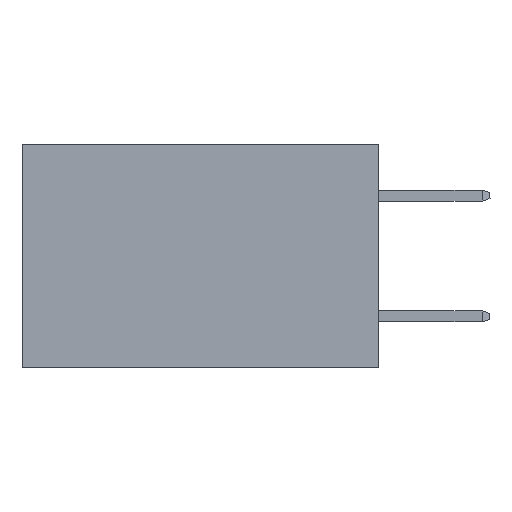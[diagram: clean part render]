
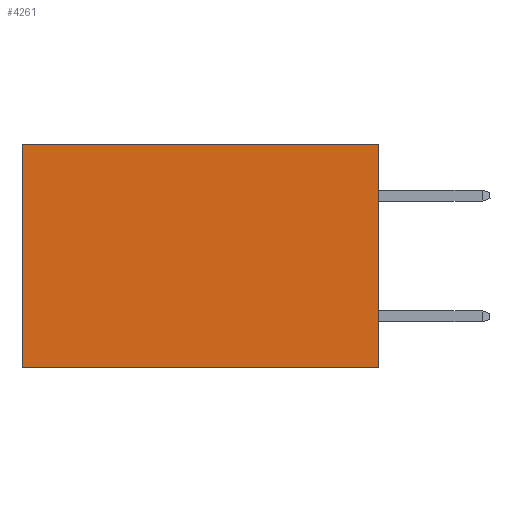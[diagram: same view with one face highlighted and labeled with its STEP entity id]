
A CAD part, left-side view. The second image highlights one B-rep face of the part: STEP entity #4261.
In plain terms, the highlighted planar face has unit normal (-1, 0, 0).
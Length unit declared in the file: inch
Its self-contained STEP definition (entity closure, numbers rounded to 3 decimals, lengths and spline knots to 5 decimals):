
#98 = DIRECTION ( 'NONE',  ( 0., 0., -1. ) ) ;
#106 = DIRECTION ( 'NONE',  ( 1., 0., 0. ) ) ;
#488 = PLANE ( 'NONE',  #5060 ) ;
#1215 = CARTESIAN_POINT ( 'NONE',  ( 0.277, 0., -0.37 ) ) ;
#1375 = DIRECTION ( 'NONE',  ( 0., 1., 0. ) ) ;
#1401 = CARTESIAN_POINT ( 'NONE',  ( 0.277, 0., 0. ) ) ;
#1468 = VECTOR ( 'NONE', #4302, 39.37008 ) ;
#1527 = EDGE_CURVE ( 'NONE', #2308, #2822, #3822, .T. ) ;
#1636 = EDGE_LOOP ( 'NONE', ( #4801, #6452, #8101, #6652 ) ) ;
#1821 = VERTEX_POINT ( 'NONE', #1215 ) ;
#1931 = DIRECTION ( 'NONE',  ( 0., 0., -1. ) ) ;
#1955 = CARTESIAN_POINT ( 'NONE',  ( 0.277, 0.59, -0.37 ) ) ;
#2147 = FACE_OUTER_BOUND ( 'NONE', #1636, .T. ) ;
#2308 = VERTEX_POINT ( 'NONE', #3587 ) ;
#2822 = VERTEX_POINT ( 'NONE', #6752 ) ;
#3281 = LINE ( 'NONE', #6185, #1468 ) ;
#3587 = CARTESIAN_POINT ( 'NONE',  ( 0.277, 0.59, 0. ) ) ;
#3822 = LINE ( 'NONE', #1955, #5441 ) ;
#4032 = DIRECTION ( 'NONE',  ( 0., 0., -1. ) ) ;
#4216 = CARTESIAN_POINT ( 'NONE',  ( 0.277, 0., -0.37 ) ) ;
#4261 = ADVANCED_FACE ( 'NONE', ( #2147 ), #488, .F. ) ;
#4302 = DIRECTION ( 'NONE',  ( 0., 1., 0. ) ) ;
#4371 = VECTOR ( 'NONE', #4032, 39.37008 ) ;
#4801 = ORIENTED_EDGE ( 'NONE', *, *, #1527, .T. ) ;
#5060 = AXIS2_PLACEMENT_3D ( 'NONE', #5841, #106, #98 ) ;
#5184 = VERTEX_POINT ( 'NONE', #5433 ) ;
#5433 = CARTESIAN_POINT ( 'NONE',  ( 0.277, 0., 0. ) ) ;
#5441 = VECTOR ( 'NONE', #1931, 39.37008 ) ;
#5760 = EDGE_CURVE ( 'NONE', #5184, #1821, #6064, .T. ) ;
#5841 = CARTESIAN_POINT ( 'NONE',  ( 0.277, 0., -0.37 ) ) ;
#6064 = LINE ( 'NONE', #4216, #4371 ) ;
#6185 = CARTESIAN_POINT ( 'NONE',  ( 0.277, 0., -0.37 ) ) ;
#6452 = ORIENTED_EDGE ( 'NONE', *, *, #8227, .F. ) ;
#6562 = EDGE_CURVE ( 'NONE', #5184, #2308, #8367, .T. ) ;
#6652 = ORIENTED_EDGE ( 'NONE', *, *, #6562, .T. ) ;
#6726 = VECTOR ( 'NONE', #1375, 39.37008 ) ;
#6752 = CARTESIAN_POINT ( 'NONE',  ( 0.277, 0.59, -0.37 ) ) ;
#8101 = ORIENTED_EDGE ( 'NONE', *, *, #5760, .F. ) ;
#8227 = EDGE_CURVE ( 'NONE', #1821, #2822, #3281, .T. ) ;
#8367 = LINE ( 'NONE', #1401, #6726 ) ;
